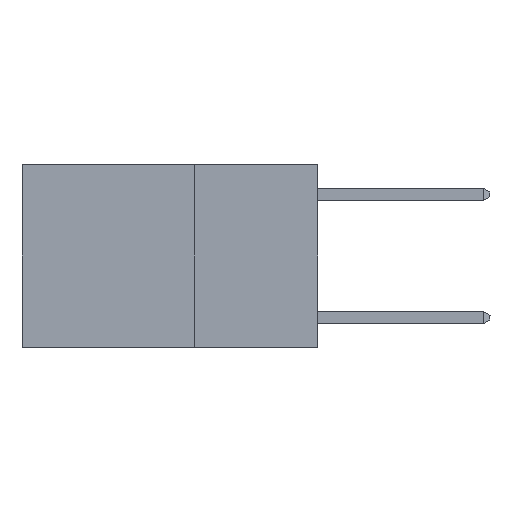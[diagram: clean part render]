
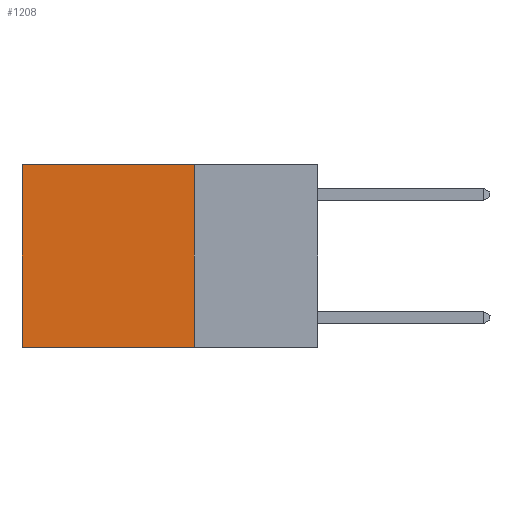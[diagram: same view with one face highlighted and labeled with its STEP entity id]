
A CAD part, left-side view. The second image highlights one B-rep face of the part: STEP entity #1208.
In plain terms, the highlighted planar face has unit normal (-1, 0, 0).
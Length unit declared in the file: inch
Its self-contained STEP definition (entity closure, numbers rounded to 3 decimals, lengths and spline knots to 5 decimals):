
#320 = EDGE_LOOP ( 'NONE', ( #8343, #12406, #13408, #3527 ) ) ;
#466 = PLANE ( 'NONE',  #11348 ) ;
#538 = CARTESIAN_POINT ( 'NONE',  ( 0.2625, 0.25, -0.37 ) ) ;
#888 = CARTESIAN_POINT ( 'NONE',  ( 0.2625, 0.25, 0. ) ) ;
#1044 = VECTOR ( 'NONE', #9114, 39.37008 ) ;
#1208 = ADVANCED_FACE ( 'NONE', ( #6598 ), #466, .F. ) ;
#2317 = EDGE_CURVE ( 'NONE', #10093, #6977, #8492, .T. ) ;
#2354 = VECTOR ( 'NONE', #11858, 39.37008 ) ;
#2513 = LINE ( 'NONE', #13395, #1044 ) ;
#2824 = VECTOR ( 'NONE', #9443, 39.37008 ) ;
#3527 = ORIENTED_EDGE ( 'NONE', *, *, #4717, .T. ) ;
#4001 = EDGE_CURVE ( 'NONE', #6111, #9435, #7890, .T. ) ;
#4629 = EDGE_CURVE ( 'NONE', #9435, #6977, #2513, .T. ) ;
#4717 = EDGE_CURVE ( 'NONE', #6111, #10093, #8499, .T. ) ;
#5253 = VECTOR ( 'NONE', #8144, 39.37008 ) ;
#6055 = CARTESIAN_POINT ( 'NONE',  ( 0.2625, 0.6, 0. ) ) ;
#6111 = VERTEX_POINT ( 'NONE', #7811 ) ;
#6598 = FACE_OUTER_BOUND ( 'NONE', #320, .T. ) ;
#6977 = VERTEX_POINT ( 'NONE', #8410 ) ;
#7811 = CARTESIAN_POINT ( 'NONE',  ( 0.2625, 0.25, 0. ) ) ;
#7890 = LINE ( 'NONE', #10823, #2354 ) ;
#7919 = DIRECTION ( 'NONE',  ( 0., 0., -1. ) ) ;
#8144 = DIRECTION ( 'NONE',  ( 0., 1., 0. ) ) ;
#8343 = ORIENTED_EDGE ( 'NONE', *, *, #2317, .T. ) ;
#8410 = CARTESIAN_POINT ( 'NONE',  ( 0.2625, 0.6, -0.37 ) ) ;
#8492 = LINE ( 'NONE', #9490, #2824 ) ;
#8499 = LINE ( 'NONE', #888, #5253 ) ;
#9114 = DIRECTION ( 'NONE',  ( 0., 1., 0. ) ) ;
#9435 = VERTEX_POINT ( 'NONE', #538 ) ;
#9443 = DIRECTION ( 'NONE',  ( 0., 0., -1. ) ) ;
#9490 = CARTESIAN_POINT ( 'NONE',  ( 0.2625, 0.6, 0. ) ) ;
#9900 = CARTESIAN_POINT ( 'NONE',  ( 0.2625, 0.25, 0. ) ) ;
#10093 = VERTEX_POINT ( 'NONE', #6055 ) ;
#10823 = CARTESIAN_POINT ( 'NONE',  ( 0.2625, 0.25, 0. ) ) ;
#11348 = AXIS2_PLACEMENT_3D ( 'NONE', #9900, #12809, #7919 ) ;
#11858 = DIRECTION ( 'NONE',  ( 0., 0., -1. ) ) ;
#12406 = ORIENTED_EDGE ( 'NONE', *, *, #4629, .F. ) ;
#12809 = DIRECTION ( 'NONE',  ( 1., 0., 0. ) ) ;
#13395 = CARTESIAN_POINT ( 'NONE',  ( 0.2625, 0.25, -0.37 ) ) ;
#13408 = ORIENTED_EDGE ( 'NONE', *, *, #4001, .F. ) ;
